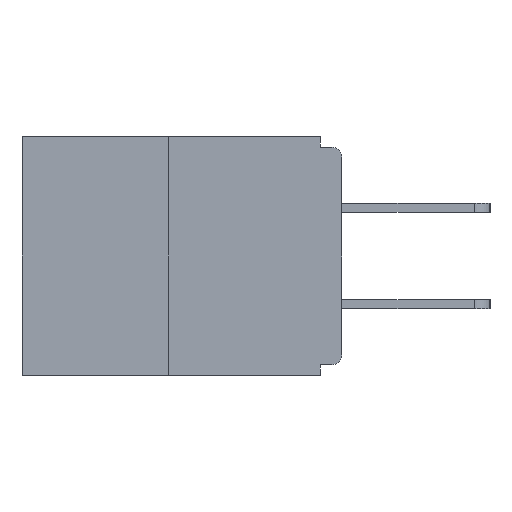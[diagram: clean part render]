
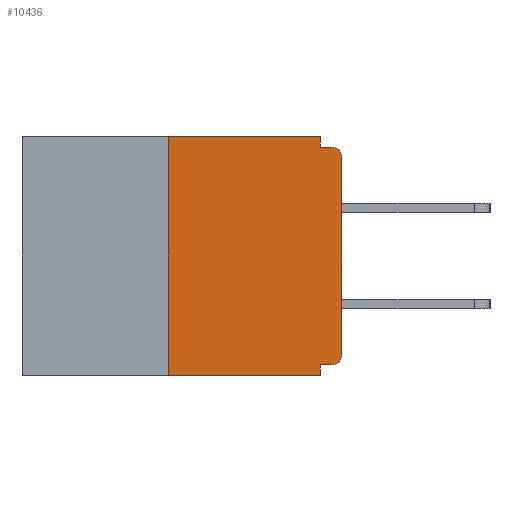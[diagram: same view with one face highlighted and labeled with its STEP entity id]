
A CAD part, left-side view. The second image highlights one B-rep face of the part: STEP entity #10436.
In plain terms, the highlighted planar face has unit normal (-1, 0, 0).
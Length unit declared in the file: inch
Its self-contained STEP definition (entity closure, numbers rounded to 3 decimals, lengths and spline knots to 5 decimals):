
#2 = ORIENTED_EDGE ( 'NONE', *, *, #1518, .F. ) ;
#38 = VECTOR ( 'NONE', #9262, 39.37008 ) ;
#128 = PLANE ( 'NONE',  #4716 ) ;
#191 = CIRCLE ( 'NONE', #2180, 0.015 ) ;
#373 = ORIENTED_EDGE ( 'NONE', *, *, #3086, .T. ) ;
#415 = DIRECTION ( 'NONE',  ( -1., 0., 0. ) ) ;
#458 = DIRECTION ( 'NONE',  ( 0., 0., -1. ) ) ;
#590 = CARTESIAN_POINT ( 'NONE',  ( 0., 0.015, -0.328 ) ) ;
#888 = ORIENTED_EDGE ( 'NONE', *, *, #3608, .T. ) ;
#1022 = VECTOR ( 'NONE', #2843, 39.37008 ) ;
#1264 = CARTESIAN_POINT ( 'NONE',  ( 0., 0.015, -0.03 ) ) ;
#1445 = DIRECTION ( 'NONE',  ( 1., 0., 0. ) ) ;
#1496 = ORIENTED_EDGE ( 'NONE', *, *, #2569, .T. ) ;
#1518 = EDGE_CURVE ( 'NONE', #10892, #3739, #4175, .T. ) ;
#2110 = ORIENTED_EDGE ( 'NONE', *, *, #10201, .F. ) ;
#2180 = AXIS2_PLACEMENT_3D ( 'NONE', #1264, #415, #458 ) ;
#2223 = VERTEX_POINT ( 'NONE', #3602 ) ;
#2353 = CARTESIAN_POINT ( 'NONE',  ( 0., 0.46, 0. ) ) ;
#2425 = VECTOR ( 'NONE', #10417, 39.37008 ) ;
#2499 = CARTESIAN_POINT ( 'NONE',  ( 0., 0.031, 0. ) ) ;
#2500 = CARTESIAN_POINT ( 'NONE',  ( 0., 0.031, -0.343 ) ) ;
#2569 = EDGE_CURVE ( 'NONE', #2223, #3739, #10329, .T. ) ;
#2768 = LINE ( 'NONE', #2812, #7144 ) ;
#2797 = LINE ( 'NONE', #10266, #38 ) ;
#2812 = CARTESIAN_POINT ( 'NONE',  ( 0., 0.031, 0. ) ) ;
#2843 = DIRECTION ( 'NONE',  ( 0., -1., 0. ) ) ;
#2987 = CARTESIAN_POINT ( 'NONE',  ( 0., 0., -0.313 ) ) ;
#3086 = EDGE_CURVE ( 'NONE', #9839, #5005, #191, .T. ) ;
#3277 = DIRECTION ( 'NONE',  ( 0., -1., 0. ) ) ;
#3345 = VERTEX_POINT ( 'NONE', #10791 ) ;
#3538 = CARTESIAN_POINT ( 'NONE',  ( 0., 0.25, 0. ) ) ;
#3602 = CARTESIAN_POINT ( 'NONE',  ( 0., 0.25, -0.343 ) ) ;
#3608 = EDGE_CURVE ( 'NONE', #4474, #11430, #11926, .T. ) ;
#3739 = VERTEX_POINT ( 'NONE', #2500 ) ;
#4175 = LINE ( 'NONE', #9358, #9747 ) ;
#4252 = EDGE_LOOP ( 'NONE', ( #8318, #2110, #1496, #2, #7121, #888, #9435, #373, #7265, #6068 ) ) ;
#4263 = AXIS2_PLACEMENT_3D ( 'NONE', #6611, #9536, #7500 ) ;
#4474 = VERTEX_POINT ( 'NONE', #590 ) ;
#4632 = EDGE_CURVE ( 'NONE', #4474, #10892, #2797, .T. ) ;
#4716 = AXIS2_PLACEMENT_3D ( 'NONE', #8863, #1445, #9907 ) ;
#4832 = VECTOR ( 'NONE', #8248, 39.37008 ) ;
#4876 = CARTESIAN_POINT ( 'NONE',  ( 0., 0., 0. ) ) ;
#5005 = VERTEX_POINT ( 'NONE', #7239 ) ;
#5098 = CARTESIAN_POINT ( 'NONE',  ( 0., 0., -0.03 ) ) ;
#5219 = LINE ( 'NONE', #4876, #2425 ) ;
#5525 = CARTESIAN_POINT ( 'NONE',  ( 0., 0., -0.015 ) ) ;
#6068 = ORIENTED_EDGE ( 'NONE', *, *, #10389, .F. ) ;
#6448 = LINE ( 'NONE', #8281, #4832 ) ;
#6611 = CARTESIAN_POINT ( 'NONE',  ( 0., 0.015, -0.313 ) ) ;
#6879 = FACE_OUTER_BOUND ( 'NONE', #4252, .T. ) ;
#7101 = EDGE_CURVE ( 'NONE', #11430, #9839, #5219, .T. ) ;
#7121 = ORIENTED_EDGE ( 'NONE', *, *, #4632, .F. ) ;
#7144 = VECTOR ( 'NONE', #11317, 39.37008 ) ;
#7239 = CARTESIAN_POINT ( 'NONE',  ( 0., 0.015, -0.015 ) ) ;
#7265 = ORIENTED_EDGE ( 'NONE', *, *, #10613, .F. ) ;
#7500 = DIRECTION ( 'NONE',  ( 0., 0., -1. ) ) ;
#7638 = LINE ( 'NONE', #2353, #8224 ) ;
#7946 = VECTOR ( 'NONE', #3277, 39.37008 ) ;
#8026 = LINE ( 'NONE', #5525, #1022 ) ;
#8224 = VECTOR ( 'NONE', #11780, 39.37008 ) ;
#8248 = DIRECTION ( 'NONE',  ( 0., 0., 1. ) ) ;
#8281 = CARTESIAN_POINT ( 'NONE',  ( 0., 0.25, 0. ) ) ;
#8318 = ORIENTED_EDGE ( 'NONE', *, *, #9716, .F. ) ;
#8863 = CARTESIAN_POINT ( 'NONE',  ( 0., 0.46, 0. ) ) ;
#8883 = CARTESIAN_POINT ( 'NONE',  ( 0., 0.46, -0.343 ) ) ;
#9262 = DIRECTION ( 'NONE',  ( 0., 1., 0. ) ) ;
#9324 = CARTESIAN_POINT ( 'NONE',  ( 0., 0.031, -0.328 ) ) ;
#9358 = CARTESIAN_POINT ( 'NONE',  ( 0., 0.031, -0.343 ) ) ;
#9435 = ORIENTED_EDGE ( 'NONE', *, *, #7101, .T. ) ;
#9524 = DIRECTION ( 'NONE',  ( 0., 0., -1. ) ) ;
#9536 = DIRECTION ( 'NONE',  ( -1., 0., 0. ) ) ;
#9716 = EDGE_CURVE ( 'NONE', #10527, #10732, #7638, .T. ) ;
#9747 = VECTOR ( 'NONE', #9524, 39.37008 ) ;
#9839 = VERTEX_POINT ( 'NONE', #5098 ) ;
#9907 = DIRECTION ( 'NONE',  ( 0., 0., -1. ) ) ;
#10201 = EDGE_CURVE ( 'NONE', #2223, #10527, #6448, .T. ) ;
#10266 = CARTESIAN_POINT ( 'NONE',  ( 0., 0., -0.328 ) ) ;
#10329 = LINE ( 'NONE', #8883, #7946 ) ;
#10389 = EDGE_CURVE ( 'NONE', #10732, #3345, #2768, .T. ) ;
#10417 = DIRECTION ( 'NONE',  ( 0., 0., 1. ) ) ;
#10436 = ADVANCED_FACE ( 'NONE', ( #6879 ), #128, .F. ) ;
#10527 = VERTEX_POINT ( 'NONE', #3538 ) ;
#10613 = EDGE_CURVE ( 'NONE', #3345, #5005, #8026, .T. ) ;
#10732 = VERTEX_POINT ( 'NONE', #2499 ) ;
#10791 = CARTESIAN_POINT ( 'NONE',  ( 0., 0.031, -0.015 ) ) ;
#10892 = VERTEX_POINT ( 'NONE', #9324 ) ;
#11317 = DIRECTION ( 'NONE',  ( 0., 0., -1. ) ) ;
#11430 = VERTEX_POINT ( 'NONE', #2987 ) ;
#11780 = DIRECTION ( 'NONE',  ( 0., -1., 0. ) ) ;
#11926 = CIRCLE ( 'NONE', #4263, 0.015 ) ;
